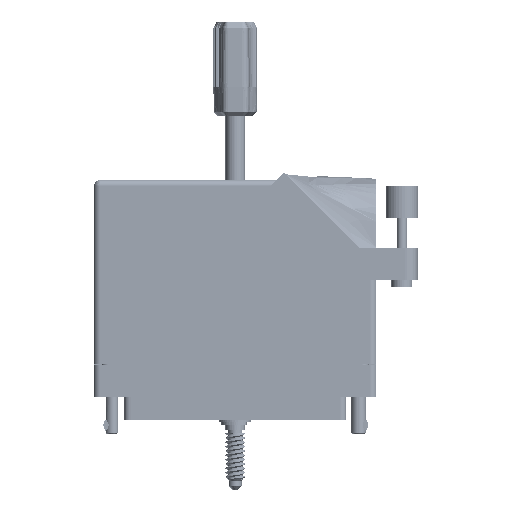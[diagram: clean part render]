
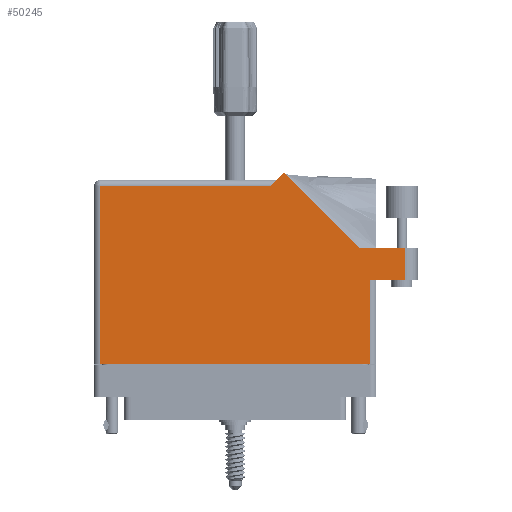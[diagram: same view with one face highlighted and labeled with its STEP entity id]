
A CAD part, front view. The second image highlights one B-rep face of the part: STEP entity #50245.
In plain terms, the highlighted face is planar.
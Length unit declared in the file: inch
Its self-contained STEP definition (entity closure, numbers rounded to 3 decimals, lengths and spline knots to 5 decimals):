
#1348 = VECTOR ( 'NONE', #55365, 39.37008 ) ;
#1932 = ORIENTED_EDGE ( 'NONE', *, *, #47769, .T. ) ;
#2197 = CARTESIAN_POINT ( 'NONE',  ( 1.359, 0.715, 0.617 ) ) ;
#2768 = VECTOR ( 'NONE', #6293, 39.37008 ) ;
#4671 = LINE ( 'NONE', #24961, #7011 ) ;
#5334 = CARTESIAN_POINT ( 'NONE',  ( -1.359, 1.613, 0.617 ) ) ;
#5831 = ORIENTED_EDGE ( 'NONE', *, *, #48927, .T. ) ;
#6085 = VERTEX_POINT ( 'NONE', #18069 ) ;
#6293 = DIRECTION ( 'NONE',  ( -1., 0., 0. ) ) ;
#7011 = VECTOR ( 'NONE', #24645, 39.37008 ) ;
#7680 = VECTOR ( 'NONE', #13801, 39.37008 ) ;
#10701 = VERTEX_POINT ( 'NONE', #38000 ) ;
#12033 = VERTEX_POINT ( 'NONE', #74327 ) ;
#13801 = DIRECTION ( 'NONE',  ( -0.707, 0.707, 0. ) ) ;
#14085 = LINE ( 'NONE', #46714, #91410 ) ;
#14510 = ORIENTED_EDGE ( 'NONE', *, *, #52072, .T. ) ;
#14669 = CARTESIAN_POINT ( 'NONE',  ( 1.634, 1.022, 0.617 ) ) ;
#15385 = VERTEX_POINT ( 'NONE', #42330 ) ;
#16494 = CARTESIAN_POINT ( 'NONE',  ( 1.634, 0.715, 0.617 ) ) ;
#18069 = CARTESIAN_POINT ( 'NONE',  ( -1.297, -0.1, 0.617 ) ) ;
#18273 = EDGE_LOOP ( 'NONE', ( #62472, #50207, #14510, #72334, #5831, #52055, #1932, #83610, #93454 ) ) ;
#20488 = VERTEX_POINT ( 'NONE', #16494 ) ;
#20987 = VERTEX_POINT ( 'NONE', #79350 ) ;
#24645 = DIRECTION ( 'NONE',  ( 1., 0., 0. ) ) ;
#24961 = CARTESIAN_POINT ( 'NONE',  ( -1.359, -0.1, 0.617 ) ) ;
#28955 = CARTESIAN_POINT ( 'NONE',  ( 1.19342, 1.022, 0.617 ) ) ;
#30156 = EDGE_CURVE ( 'NONE', #10701, #15385, #46109, .T. ) ;
#30876 = CARTESIAN_POINT ( 'NONE',  ( -1.359, 1.675, 0.617 ) ) ;
#33525 = VERTEX_POINT ( 'NONE', #46236 ) ;
#37116 = CARTESIAN_POINT ( 'NONE',  ( -1.297, -0.1, 0.617 ) ) ;
#37256 = DIRECTION ( 'NONE',  ( -1., 0., 0. ) ) ;
#38000 = CARTESIAN_POINT ( 'NONE',  ( 1.297, -0.1, 0.617 ) ) ;
#39149 = DIRECTION ( 'NONE',  ( -0.707, -0.707, 0. ) ) ;
#39166 = LINE ( 'NONE', #5334, #2768 ) ;
#40826 = CARTESIAN_POINT ( 'NONE',  ( 1.297, 0.715, 0.617 ) ) ;
#42330 = CARTESIAN_POINT ( 'NONE',  ( 1.297, 0.715, 0.617 ) ) ;
#43659 = VERTEX_POINT ( 'NONE', #14669 ) ;
#46109 = LINE ( 'NONE', #40826, #62510 ) ;
#46236 = CARTESIAN_POINT ( 'NONE',  ( 0.337, 1.613, 0.617 ) ) ;
#46714 = CARTESIAN_POINT ( 'NONE',  ( 0.399, 1.675, 0.617 ) ) ;
#47769 = EDGE_CURVE ( 'NONE', #91437, #6085, #70577, .T. ) ;
#48927 = EDGE_CURVE ( 'NONE', #12033, #33525, #14085, .T. ) ;
#50207 = ORIENTED_EDGE ( 'NONE', *, *, #86934, .T. ) ;
#50245 = ADVANCED_FACE ( 'NONE', ( #86502 ), #75648, .F. ) ;
#51133 = VECTOR ( 'NONE', #37256, 39.37008 ) ;
#52055 = ORIENTED_EDGE ( 'NONE', *, *, #58625, .T. ) ;
#52072 = EDGE_CURVE ( 'NONE', #43659, #20987, #61605, .T. ) ;
#55365 = DIRECTION ( 'NONE',  ( 0., 1., 0. ) ) ;
#58550 = LINE ( 'NONE', #2197, #87779 ) ;
#58625 = EDGE_CURVE ( 'NONE', #33525, #91437, #39166, .T. ) ;
#59127 = AXIS2_PLACEMENT_3D ( 'NONE', #30876, #83104, #93249 ) ;
#59827 = CARTESIAN_POINT ( 'NONE',  ( 1.759, 1.022, 0.617 ) ) ;
#61605 = LINE ( 'NONE', #59827, #51133 ) ;
#62472 = ORIENTED_EDGE ( 'NONE', *, *, #64494, .T. ) ;
#62510 = VECTOR ( 'NONE', #70913, 39.37008 ) ;
#62772 = LINE ( 'NONE', #28955, #7680 ) ;
#64102 = EDGE_CURVE ( 'NONE', #6085, #10701, #4671, .T. ) ;
#64494 = EDGE_CURVE ( 'NONE', #15385, #20488, #58550, .T. ) ;
#64852 = CARTESIAN_POINT ( 'NONE',  ( 1.634, 1.022, 0.617 ) ) ;
#69273 = LINE ( 'NONE', #64852, #1348 ) ;
#70577 = LINE ( 'NONE', #37116, #83365 ) ;
#70913 = DIRECTION ( 'NONE',  ( 0., 1., 0. ) ) ;
#72334 = ORIENTED_EDGE ( 'NONE', *, *, #84185, .T. ) ;
#74327 = CARTESIAN_POINT ( 'NONE',  ( 0.46971, 1.74571, 0.617 ) ) ;
#75648 = PLANE ( 'NONE',  #59127 ) ;
#79350 = CARTESIAN_POINT ( 'NONE',  ( 1.19342, 1.022, 0.617 ) ) ;
#82496 = DIRECTION ( 'NONE',  ( 0., -1., 0. ) ) ;
#83104 = DIRECTION ( 'NONE',  ( 0., 0., -1. ) ) ;
#83365 = VECTOR ( 'NONE', #82496, 39.37008 ) ;
#83610 = ORIENTED_EDGE ( 'NONE', *, *, #64102, .T. ) ;
#84185 = EDGE_CURVE ( 'NONE', #20987, #12033, #62772, .T. ) ;
#84617 = DIRECTION ( 'NONE',  ( 1., 0., 0. ) ) ;
#86502 = FACE_OUTER_BOUND ( 'NONE', #18273, .T. ) ;
#86934 = EDGE_CURVE ( 'NONE', #20488, #43659, #69273, .T. ) ;
#87779 = VECTOR ( 'NONE', #84617, 39.37008 ) ;
#91410 = VECTOR ( 'NONE', #39149, 39.37008 ) ;
#91437 = VERTEX_POINT ( 'NONE', #91996 ) ;
#91996 = CARTESIAN_POINT ( 'NONE',  ( -1.297, 1.613, 0.617 ) ) ;
#93249 = DIRECTION ( 'NONE',  ( -1., 0., 0. ) ) ;
#93454 = ORIENTED_EDGE ( 'NONE', *, *, #30156, .T. ) ;
